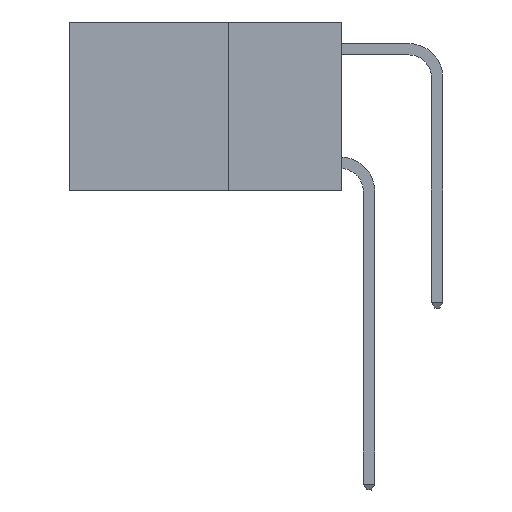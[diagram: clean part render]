
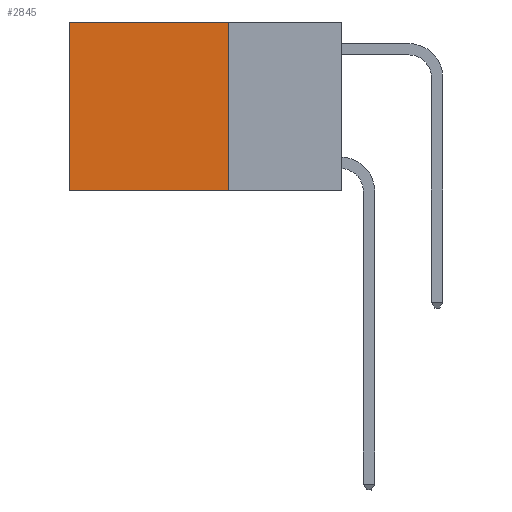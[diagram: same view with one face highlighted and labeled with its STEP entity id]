
A CAD part, left-side view. The second image highlights one B-rep face of the part: STEP entity #2845.
In plain terms, the highlighted planar face has unit normal (-1, 0, 0).
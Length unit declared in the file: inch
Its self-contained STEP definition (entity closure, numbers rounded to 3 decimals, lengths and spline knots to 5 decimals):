
#1138 = AXIS2_PLACEMENT_3D ( 'NONE', #22578, #14522, #2841 ) ;
#1188 = EDGE_LOOP ( 'NONE', ( #6997, #24407, #16678, #22679 ) ) ;
#1895 = LINE ( 'NONE', #20159, #9115 ) ;
#2260 = DIRECTION ( 'NONE',  ( 0., 1., 0. ) ) ;
#2841 = DIRECTION ( 'NONE',  ( 0., 0., -1. ) ) ;
#2845 = ADVANCED_FACE ( 'NONE', ( #12921 ), #16768, .F. ) ;
#3647 = CARTESIAN_POINT ( 'NONE',  ( 0.2625, 0.6, -0.37 ) ) ;
#4041 = DIRECTION ( 'NONE',  ( 0., 0., -1. ) ) ;
#5336 = CARTESIAN_POINT ( 'NONE',  ( 0.2625, 0.25, -0.37 ) ) ;
#6474 = VECTOR ( 'NONE', #13100, 39.37008 ) ;
#6505 = EDGE_CURVE ( 'NONE', #18977, #16894, #24742, .T. ) ;
#6997 = ORIENTED_EDGE ( 'NONE', *, *, #14400, .T. ) ;
#7440 = LINE ( 'NONE', #5336, #24919 ) ;
#9115 = VECTOR ( 'NONE', #4041, 39.37008 ) ;
#10236 = VECTOR ( 'NONE', #2260, 39.37008 ) ;
#10758 = CARTESIAN_POINT ( 'NONE',  ( 0.2625, 0.25, 0. ) ) ;
#11402 = DIRECTION ( 'NONE',  ( 0., 1., 0. ) ) ;
#12712 = CARTESIAN_POINT ( 'NONE',  ( 0.2625, 0.25, 0. ) ) ;
#12921 = FACE_OUTER_BOUND ( 'NONE', #1188, .T. ) ;
#13100 = DIRECTION ( 'NONE',  ( 0., 0., -1. ) ) ;
#14400 = EDGE_CURVE ( 'NONE', #16894, #21308, #15104, .T. ) ;
#14522 = DIRECTION ( 'NONE',  ( 1., 0., 0. ) ) ;
#15104 = LINE ( 'NONE', #23149, #6474 ) ;
#15419 = CARTESIAN_POINT ( 'NONE',  ( 0.2625, 0.25, -0.37 ) ) ;
#15845 = CARTESIAN_POINT ( 'NONE',  ( 0.2625, 0.6, 0. ) ) ;
#16678 = ORIENTED_EDGE ( 'NONE', *, *, #18796, .F. ) ;
#16768 = PLANE ( 'NONE',  #1138 ) ;
#16894 = VERTEX_POINT ( 'NONE', #15845 ) ;
#18796 = EDGE_CURVE ( 'NONE', #18977, #20054, #1895, .T. ) ;
#18977 = VERTEX_POINT ( 'NONE', #10758 ) ;
#20054 = VERTEX_POINT ( 'NONE', #15419 ) ;
#20159 = CARTESIAN_POINT ( 'NONE',  ( 0.2625, 0.25, 0. ) ) ;
#21308 = VERTEX_POINT ( 'NONE', #3647 ) ;
#22553 = EDGE_CURVE ( 'NONE', #20054, #21308, #7440, .T. ) ;
#22578 = CARTESIAN_POINT ( 'NONE',  ( 0.2625, 0.25, 0. ) ) ;
#22679 = ORIENTED_EDGE ( 'NONE', *, *, #6505, .T. ) ;
#23149 = CARTESIAN_POINT ( 'NONE',  ( 0.2625, 0.6, 0. ) ) ;
#24407 = ORIENTED_EDGE ( 'NONE', *, *, #22553, .F. ) ;
#24742 = LINE ( 'NONE', #12712, #10236 ) ;
#24919 = VECTOR ( 'NONE', #11402, 39.37008 ) ;
